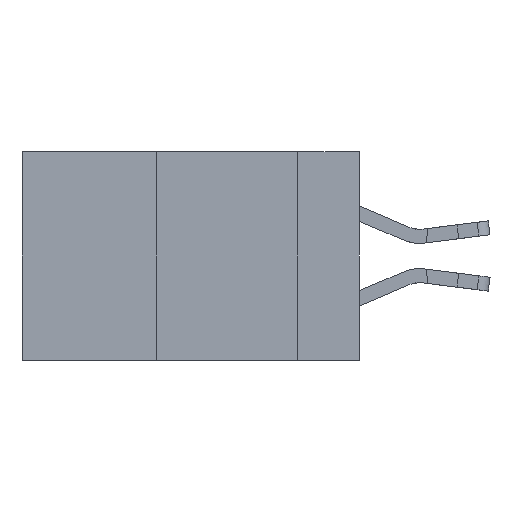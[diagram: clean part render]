
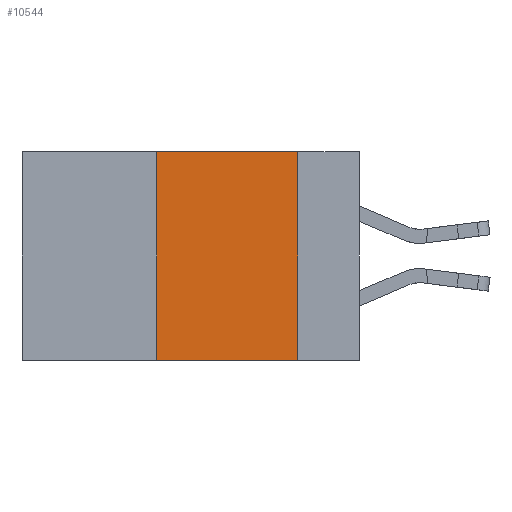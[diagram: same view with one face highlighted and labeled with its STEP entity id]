
A CAD part, left-side view. The second image highlights one B-rep face of the part: STEP entity #10544.
In plain terms, the highlighted planar face has unit normal (-1, 0, 0).
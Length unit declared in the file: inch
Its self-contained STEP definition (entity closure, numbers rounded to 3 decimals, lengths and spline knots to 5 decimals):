
#756 = CARTESIAN_POINT ( 'NONE',  ( 0., 0.11, 0. ) ) ;
#1418 = DIRECTION ( 'NONE',  ( 0., 0., 1. ) ) ;
#1648 = AXIS2_PLACEMENT_3D ( 'NONE', #6350, #8402, #15922 ) ;
#2013 = EDGE_CURVE ( 'NONE', #5458, #4710, #17051, .T. ) ;
#2100 = VECTOR ( 'NONE', #19378, 39.37008 ) ;
#3043 = CARTESIAN_POINT ( 'NONE',  ( 0., 0.36, -0.37 ) ) ;
#3535 = VECTOR ( 'NONE', #8098, 39.37008 ) ;
#3610 = EDGE_CURVE ( 'NONE', #10649, #4710, #24007, .T. ) ;
#4193 = VERTEX_POINT ( 'NONE', #8282 ) ;
#4710 = VERTEX_POINT ( 'NONE', #11197 ) ;
#5327 = ORIENTED_EDGE ( 'NONE', *, *, #16266, .F. ) ;
#5458 = VERTEX_POINT ( 'NONE', #16903 ) ;
#5773 = FACE_OUTER_BOUND ( 'NONE', #15438, .T. ) ;
#6171 = CARTESIAN_POINT ( 'NONE',  ( 0., 0.6, -0.37 ) ) ;
#6350 = CARTESIAN_POINT ( 'NONE',  ( 0., 0.6, 0. ) ) ;
#8098 = DIRECTION ( 'NONE',  ( 0., 0., -1. ) ) ;
#8282 = CARTESIAN_POINT ( 'NONE',  ( 0., 0.36, 0. ) ) ;
#8402 = DIRECTION ( 'NONE',  ( 1., 0., 0. ) ) ;
#9252 = CARTESIAN_POINT ( 'NONE',  ( 0., 0.36, 0. ) ) ;
#9426 = LINE ( 'NONE', #9252, #11443 ) ;
#10216 = VECTOR ( 'NONE', #22647, 39.37008 ) ;
#10544 = ADVANCED_FACE ( 'NONE', ( #5773 ), #12152, .F. ) ;
#10649 = VERTEX_POINT ( 'NONE', #3043 ) ;
#11197 = CARTESIAN_POINT ( 'NONE',  ( 0., 0.11, -0.37 ) ) ;
#11443 = VECTOR ( 'NONE', #1418, 39.37008 ) ;
#11741 = CARTESIAN_POINT ( 'NONE',  ( 0., 0.6, 0. ) ) ;
#11768 = LINE ( 'NONE', #11741, #2100 ) ;
#12152 = PLANE ( 'NONE',  #1648 ) ;
#15438 = EDGE_LOOP ( 'NONE', ( #22760, #18555, #5327, #16393 ) ) ;
#15922 = DIRECTION ( 'NONE',  ( 0., 0., -1. ) ) ;
#16266 = EDGE_CURVE ( 'NONE', #10649, #4193, #9426, .T. ) ;
#16393 = ORIENTED_EDGE ( 'NONE', *, *, #3610, .T. ) ;
#16903 = CARTESIAN_POINT ( 'NONE',  ( 0., 0.11, 0. ) ) ;
#17051 = LINE ( 'NONE', #756, #3535 ) ;
#18555 = ORIENTED_EDGE ( 'NONE', *, *, #19185, .F. ) ;
#19185 = EDGE_CURVE ( 'NONE', #4193, #5458, #11768, .T. ) ;
#19378 = DIRECTION ( 'NONE',  ( 0., -1., 0. ) ) ;
#22647 = DIRECTION ( 'NONE',  ( 0., -1., 0. ) ) ;
#22760 = ORIENTED_EDGE ( 'NONE', *, *, #2013, .F. ) ;
#24007 = LINE ( 'NONE', #6171, #10216 ) ;
